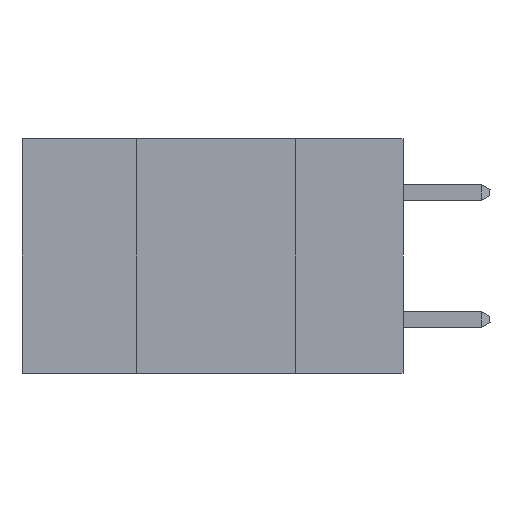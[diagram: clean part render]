
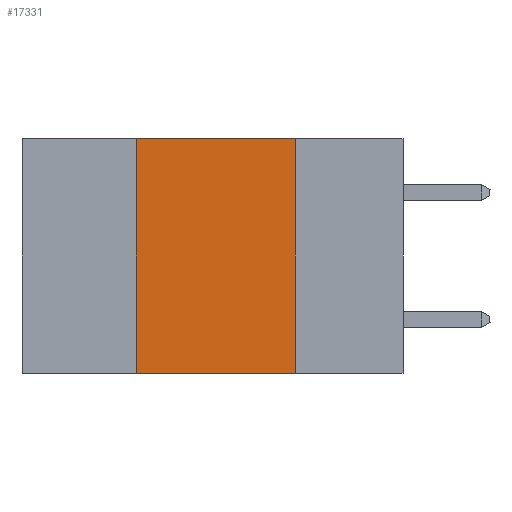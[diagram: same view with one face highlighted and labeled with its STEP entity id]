
A CAD part, left-side view. The second image highlights one B-rep face of the part: STEP entity #17331.
In plain terms, the highlighted planar face has unit normal (-1, 0, 0).
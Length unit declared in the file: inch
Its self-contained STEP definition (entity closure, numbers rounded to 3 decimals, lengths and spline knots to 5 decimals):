
#632 = EDGE_CURVE ( 'NONE', #31790, #27909, #6578, .T. ) ;
#2339 = ORIENTED_EDGE ( 'NONE', *, *, #39499, .F. ) ;
#4264 = VECTOR ( 'NONE', #24535, 39.37008 ) ;
#6578 = LINE ( 'NONE', #9818, #4264 ) ;
#7527 = LINE ( 'NONE', #39536, #42307 ) ;
#7852 = EDGE_CURVE ( 'NONE', #31790, #11548, #27173, .T. ) ;
#9818 = CARTESIAN_POINT ( 'NONE',  ( 0., 0.6, -0.37 ) ) ;
#11548 = VERTEX_POINT ( 'NONE', #14149 ) ;
#12411 = LINE ( 'NONE', #14108, #13556 ) ;
#13015 = CARTESIAN_POINT ( 'NONE',  ( 0., 0.17, 0. ) ) ;
#13556 = VECTOR ( 'NONE', #39594, 39.37008 ) ;
#14108 = CARTESIAN_POINT ( 'NONE',  ( 0., 0.17, 0. ) ) ;
#14149 = CARTESIAN_POINT ( 'NONE',  ( 0., 0.42, 0. ) ) ;
#14231 = CARTESIAN_POINT ( 'NONE',  ( 0., 0.6, 0. ) ) ;
#17331 = ADVANCED_FACE ( 'NONE', ( #17534 ), #17787, .F. ) ;
#17534 = FACE_OUTER_BOUND ( 'NONE', #17699, .T. ) ;
#17699 = EDGE_LOOP ( 'NONE', ( #2339, #36476, #32258, #18072 ) ) ;
#17787 = PLANE ( 'NONE',  #40793 ) ;
#18072 = ORIENTED_EDGE ( 'NONE', *, *, #632, .T. ) ;
#21472 = CARTESIAN_POINT ( 'NONE',  ( 0., 0.42, 0. ) ) ;
#22146 = CARTESIAN_POINT ( 'NONE',  ( 0., 0.17, -0.37 ) ) ;
#22619 = CARTESIAN_POINT ( 'NONE',  ( 0., 0.42, -0.37 ) ) ;
#24535 = DIRECTION ( 'NONE',  ( 0., -1., 0. ) ) ;
#27173 = LINE ( 'NONE', #21472, #42263 ) ;
#27909 = VERTEX_POINT ( 'NONE', #22146 ) ;
#28654 = DIRECTION ( 'NONE',  ( 0., 0., -1. ) ) ;
#30101 = VERTEX_POINT ( 'NONE', #13015 ) ;
#31790 = VERTEX_POINT ( 'NONE', #22619 ) ;
#32232 = DIRECTION ( 'NONE',  ( 1., 0., 0. ) ) ;
#32258 = ORIENTED_EDGE ( 'NONE', *, *, #7852, .F. ) ;
#36476 = ORIENTED_EDGE ( 'NONE', *, *, #42546, .F. ) ;
#39499 = EDGE_CURVE ( 'NONE', #30101, #27909, #12411, .T. ) ;
#39536 = CARTESIAN_POINT ( 'NONE',  ( 0., 0.6, 0. ) ) ;
#39594 = DIRECTION ( 'NONE',  ( 0., 0., -1. ) ) ;
#40793 = AXIS2_PLACEMENT_3D ( 'NONE', #14231, #32232, #28654 ) ;
#42263 = VECTOR ( 'NONE', #44347, 39.37008 ) ;
#42307 = VECTOR ( 'NONE', #46622, 39.37008 ) ;
#42546 = EDGE_CURVE ( 'NONE', #11548, #30101, #7527, .T. ) ;
#44347 = DIRECTION ( 'NONE',  ( 0., 0., 1. ) ) ;
#46622 = DIRECTION ( 'NONE',  ( 0., -1., 0. ) ) ;
